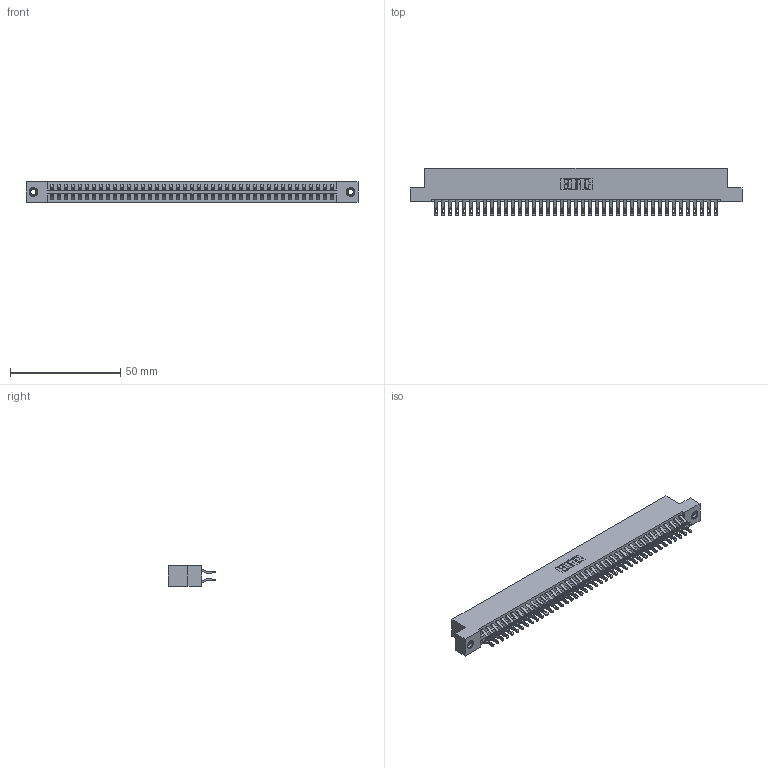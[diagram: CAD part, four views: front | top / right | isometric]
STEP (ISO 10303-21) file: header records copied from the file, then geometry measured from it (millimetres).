
FILE_DESCRIPTION (( 'STEP AP203' ), '1' );
FILE_NAME ('346-082-555-207.STEP', '2022-05-25T18:12:09', ( '' ), ( '' ), 'SwSTEP 2.0', 'SolidWorks 2020', '' );
FILE_SCHEMA (( 'CONFIG_CONTROL_DESIGN' ));
Length unit declared in the file: inch
Products named in the file (4): 345-250-001_345-250-005-103; 346 Part_Flush Mounting Lugs - 0.156 Dia-TI; 346-082-555-207; 345-292-001_555 Tail
Assembly tree (85 placements, depth 2):
  346-082-555-207
    346 Part_Flush Mounting Lugs - 0.156 Dia-TI
    345-292-001_555 Tail  x82
    345-250-001_345-250-005-103  x2
Bounding box: 150.75 x 21.46 x 9.4 mm (x, y, z)
Volume: 14916.5 mm3; surface area: 21369.5 mm2
Topology: 85 solids, 85 shells, 4938 faces, 15471 edges, 10306 vertices
Faces by surface type: plane 2814, cylinder 2108, cone 12, torus 4
Entity records: 28404 total; most frequent: CARTESIAN_POINT 4701, ORIENTED_EDGE 4598, DIRECTION 4189, EDGE_CURVE 2299, LINE 1963, VECTOR 1963, VERTEX_POINT 1528, AXIS2_PLACEMENT_3D 1113
